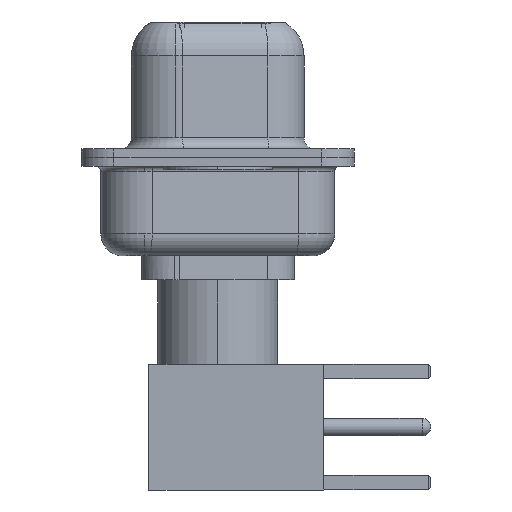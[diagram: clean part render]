
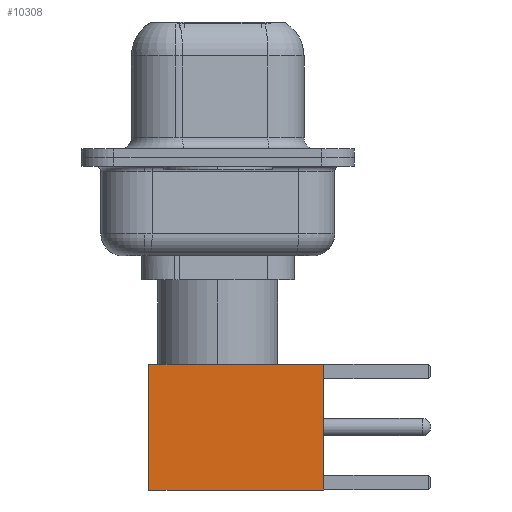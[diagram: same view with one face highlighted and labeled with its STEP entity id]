
A CAD part, left-side view. The second image highlights one B-rep face of the part: STEP entity #10308.
In plain terms, the highlighted face is planar.
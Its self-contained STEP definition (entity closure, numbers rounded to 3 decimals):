
#9 = CARTESIAN_POINT ( 'NONE',  ( -2.875, 2.875, 8. ) ) ;
#375 = EDGE_CURVE ( 'NONE', #15759, #6042, #9729, .T. ) ;
#1049 = EDGE_CURVE ( 'NONE', #2101, #15403, #1420, .T. ) ;
#1378 = CARTESIAN_POINT ( 'NONE',  ( 2.875, 2.875, 0. ) ) ;
#1420 = LINE ( 'NONE', #3020, #1644 ) ;
#1451 = PLANE ( 'NONE',  #2374 ) ;
#1617 = LINE ( 'NONE', #12902, #15779 ) ;
#1621 = DIRECTION ( 'NONE',  ( 0., 1., 0. ) ) ;
#1644 = VECTOR ( 'NONE', #11908, 1000. ) ;
#2101 = VERTEX_POINT ( 'NONE', #13191 ) ;
#2253 = EDGE_LOOP ( 'NONE', ( #11633, #2407, #12752, #9875 ) ) ;
#2374 = AXIS2_PLACEMENT_3D ( 'NONE', #1378, #1621, #9348 ) ;
#2407 = ORIENTED_EDGE ( 'NONE', *, *, #375, .T. ) ;
#2532 = LINE ( 'NONE', #11159, #9389 ) ;
#3020 = CARTESIAN_POINT ( 'NONE',  ( 0., 2.875, 8. ) ) ;
#5877 = CARTESIAN_POINT ( 'NONE',  ( -2.875, 2.875, 0. ) ) ;
#6042 = VERTEX_POINT ( 'NONE', #5877 ) ;
#9348 = DIRECTION ( 'NONE',  ( 0., 0., 1. ) ) ;
#9389 = VECTOR ( 'NONE', #15179, 1000. ) ;
#9492 = CARTESIAN_POINT ( 'NONE',  ( 2.875, 2.875, 0. ) ) ;
#9729 = LINE ( 'NONE', #14823, #12152 ) ;
#9875 = ORIENTED_EDGE ( 'NONE', *, *, #1049, .F. ) ;
#10308 = ADVANCED_FACE ( 'NONE', ( #14451 ), #1451, .T. ) ;
#11159 = CARTESIAN_POINT ( 'NONE',  ( 2.875, 2.875, 0. ) ) ;
#11403 = EDGE_CURVE ( 'NONE', #15403, #6042, #1617, .T. ) ;
#11633 = ORIENTED_EDGE ( 'NONE', *, *, #15434, .T. ) ;
#11703 = DIRECTION ( 'NONE',  ( -1., 0., 0. ) ) ;
#11908 = DIRECTION ( 'NONE',  ( -1., 0., 0. ) ) ;
#12152 = VECTOR ( 'NONE', #11703, 1000. ) ;
#12752 = ORIENTED_EDGE ( 'NONE', *, *, #11403, .F. ) ;
#12902 = CARTESIAN_POINT ( 'NONE',  ( -2.875, 2.875, 0. ) ) ;
#13191 = CARTESIAN_POINT ( 'NONE',  ( 2.875, 2.875, 8. ) ) ;
#14249 = DIRECTION ( 'NONE',  ( 0., 0., -1. ) ) ;
#14451 = FACE_OUTER_BOUND ( 'NONE', #2253, .T. ) ;
#14823 = CARTESIAN_POINT ( 'NONE',  ( 0., 2.875, 0. ) ) ;
#15179 = DIRECTION ( 'NONE',  ( 0., 0., -1. ) ) ;
#15403 = VERTEX_POINT ( 'NONE', #9 ) ;
#15434 = EDGE_CURVE ( 'NONE', #2101, #15759, #2532, .T. ) ;
#15759 = VERTEX_POINT ( 'NONE', #9492 ) ;
#15779 = VECTOR ( 'NONE', #14249, 1000. ) ;
